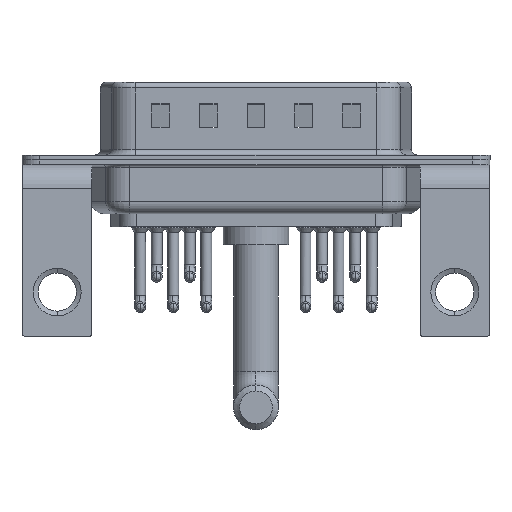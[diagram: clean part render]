
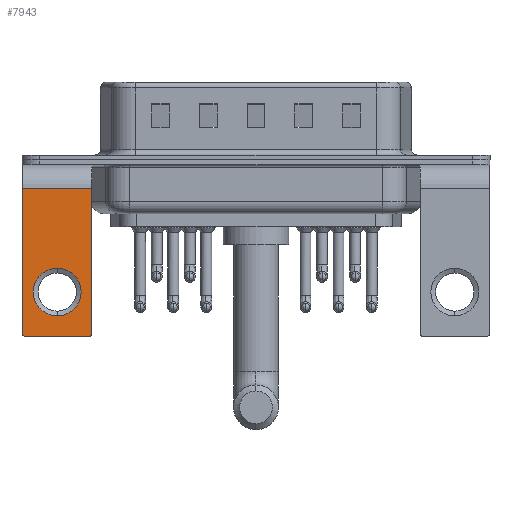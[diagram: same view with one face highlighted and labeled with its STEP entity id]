
A CAD part, front view. The second image highlights one B-rep face of the part: STEP entity #7943.
In plain terms, the highlighted planar face has unit normal (0, -1, 0).
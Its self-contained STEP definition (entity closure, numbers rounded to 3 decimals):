
#230 = CARTESIAN_POINT ( 'NONE',  ( 2.9, -6.25, -14.8 ) ) ;
#699 = DIRECTION ( 'NONE',  ( 0., 0., -1. ) ) ;
#1051 = CARTESIAN_POINT ( 'NONE',  ( -2.65, -6.25, -14.55 ) ) ;
#1276 = CARTESIAN_POINT ( 'NONE',  ( 2.9, -6.25, -2.4 ) ) ;
#2115 = LINE ( 'NONE', #2465, #7643 ) ;
#2271 = DIRECTION ( 'NONE',  ( 0., 0., -1. ) ) ;
#2465 = CARTESIAN_POINT ( 'NONE',  ( 2.9, -6.25, -2.4 ) ) ;
#2537 = EDGE_CURVE ( 'NONE', #18426, #9524, #23226, .T. ) ;
#2620 = CARTESIAN_POINT ( 'NONE',  ( -2.9, -6.25, -2.4 ) ) ;
#2639 = CARTESIAN_POINT ( 'NONE',  ( 2.65, -6.25, -14.55 ) ) ;
#3290 = EDGE_CURVE ( 'NONE', #13451, #18426, #9300, .T. ) ;
#3456 = ORIENTED_EDGE ( 'NONE', *, *, #14686, .F. ) ;
#3663 = ORIENTED_EDGE ( 'NONE', *, *, #17173, .F. ) ;
#4831 = CARTESIAN_POINT ( 'NONE',  ( 0., -6.25, -13.07 ) ) ;
#4839 = CARTESIAN_POINT ( 'NONE',  ( 2.9, -6.25, -2.4 ) ) ;
#4960 = ORIENTED_EDGE ( 'NONE', *, *, #17511, .T. ) ;
#5236 = AXIS2_PLACEMENT_3D ( 'NONE', #21547, #9016, #12682 ) ;
#5382 = DIRECTION ( 'NONE',  ( -1., 0., 0. ) ) ;
#5528 = LINE ( 'NONE', #230, #9959 ) ;
#5682 = VERTEX_POINT ( 'NONE', #4831 ) ;
#6343 = DIRECTION ( 'NONE',  ( 0., 0., 1. ) ) ;
#6499 = DIRECTION ( 'NONE',  ( 0., -1., 0. ) ) ;
#6607 = ORIENTED_EDGE ( 'NONE', *, *, #22236, .T. ) ;
#7570 = CARTESIAN_POINT ( 'NONE',  ( -2.65, -6.25, -14.8 ) ) ;
#7643 = VECTOR ( 'NONE', #699, 1000. ) ;
#7943 = ADVANCED_FACE ( 'NONE', ( #17419, #9273 ), #16475, .F. ) ;
#8417 = EDGE_LOOP ( 'NONE', ( #12990, #19633, #3663, #22960, #3456, #4960 ) ) ;
#8478 = EDGE_LOOP ( 'NONE', ( #6607, #13731 ) ) ;
#8904 = VERTEX_POINT ( 'NONE', #14419 ) ;
#9016 = DIRECTION ( 'NONE',  ( 0., 1., 0. ) ) ;
#9037 = CARTESIAN_POINT ( 'NONE',  ( 2.9, -6.25, -2.4 ) ) ;
#9273 = FACE_OUTER_BOUND ( 'NONE', #8417, .T. ) ;
#9300 = LINE ( 'NONE', #2620, #22711 ) ;
#9524 = VERTEX_POINT ( 'NONE', #7570 ) ;
#9624 = EDGE_CURVE ( 'NONE', #14152, #23138, #21000, .T. ) ;
#9945 = DIRECTION ( 'NONE',  ( 0., 0., 1. ) ) ;
#9959 = VECTOR ( 'NONE', #12830, 1000. ) ;
#10200 = LINE ( 'NONE', #1276, #21317 ) ;
#11499 = CIRCLE ( 'NONE', #19087, 2. ) ;
#11632 = DIRECTION ( 'NONE',  ( 0., -1., 0. ) ) ;
#12682 = DIRECTION ( 'NONE',  ( 0., 0., 1. ) ) ;
#12827 = DIRECTION ( 'NONE',  ( 0., 1., 0. ) ) ;
#12830 = DIRECTION ( 'NONE',  ( -1., 0., 0. ) ) ;
#12928 = CARTESIAN_POINT ( 'NONE',  ( 2.65, -6.25, -14.8 ) ) ;
#12990 = ORIENTED_EDGE ( 'NONE', *, *, #3290, .T. ) ;
#13451 = VERTEX_POINT ( 'NONE', #20662 ) ;
#13731 = ORIENTED_EDGE ( 'NONE', *, *, #19025, .T. ) ;
#14152 = VERTEX_POINT ( 'NONE', #12928 ) ;
#14419 = CARTESIAN_POINT ( 'NONE',  ( 0., -6.25, -9.07 ) ) ;
#14686 = EDGE_CURVE ( 'NONE', #20490, #23138, #2115, .T. ) ;
#16038 = CARTESIAN_POINT ( 'NONE',  ( 2.9, -6.25, -14.55 ) ) ;
#16374 = AXIS2_PLACEMENT_3D ( 'NONE', #9037, #12827, #18004 ) ;
#16475 = PLANE ( 'NONE',  #16374 ) ;
#16843 = AXIS2_PLACEMENT_3D ( 'NONE', #2639, #6499, #22784 ) ;
#17173 = EDGE_CURVE ( 'NONE', #14152, #9524, #5528, .T. ) ;
#17419 = FACE_BOUND ( 'NONE', #8478, .T. ) ;
#17511 = EDGE_CURVE ( 'NONE', #20490, #13451, #10200, .T. ) ;
#17907 = AXIS2_PLACEMENT_3D ( 'NONE', #1051, #11632, #6343 ) ;
#18004 = DIRECTION ( 'NONE',  ( 0., 0., 1. ) ) ;
#18426 = VERTEX_POINT ( 'NONE', #19827 ) ;
#18820 = CARTESIAN_POINT ( 'NONE',  ( 0., -6.25, -11.07 ) ) ;
#19025 = EDGE_CURVE ( 'NONE', #8904, #5682, #11499, .T. ) ;
#19087 = AXIS2_PLACEMENT_3D ( 'NONE', #18820, #20715, #9945 ) ;
#19633 = ORIENTED_EDGE ( 'NONE', *, *, #2537, .T. ) ;
#19827 = CARTESIAN_POINT ( 'NONE',  ( -2.9, -6.25, -14.55 ) ) ;
#20300 = CIRCLE ( 'NONE', #5236, 2. ) ;
#20490 = VERTEX_POINT ( 'NONE', #4839 ) ;
#20662 = CARTESIAN_POINT ( 'NONE',  ( -2.9, -6.25, -2.4 ) ) ;
#20715 = DIRECTION ( 'NONE',  ( 0., 1., 0. ) ) ;
#21000 = CIRCLE ( 'NONE', #16843, 0.25 ) ;
#21317 = VECTOR ( 'NONE', #5382, 1000. ) ;
#21547 = CARTESIAN_POINT ( 'NONE',  ( 0., -6.25, -11.07 ) ) ;
#22236 = EDGE_CURVE ( 'NONE', #5682, #8904, #20300, .T. ) ;
#22711 = VECTOR ( 'NONE', #2271, 1000. ) ;
#22784 = DIRECTION ( 'NONE',  ( 0., 0., 1. ) ) ;
#22960 = ORIENTED_EDGE ( 'NONE', *, *, #9624, .T. ) ;
#23138 = VERTEX_POINT ( 'NONE', #16038 ) ;
#23226 = CIRCLE ( 'NONE', #17907, 0.25 ) ;
